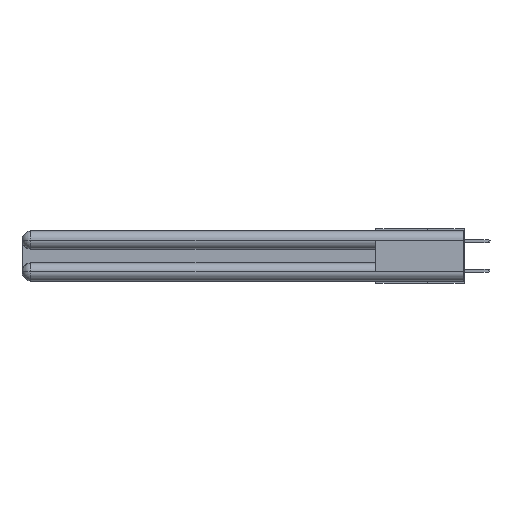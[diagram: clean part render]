
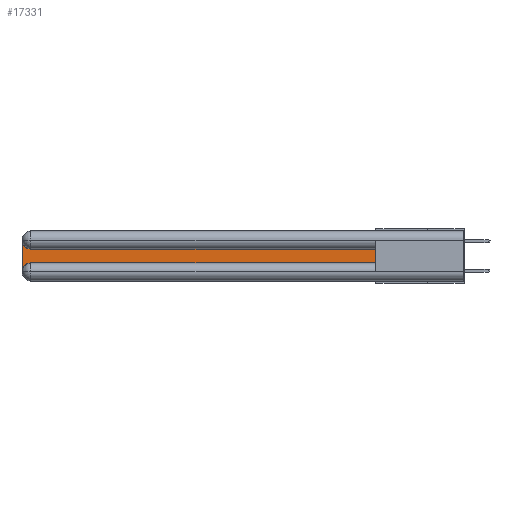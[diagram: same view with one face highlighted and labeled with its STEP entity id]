
A CAD part, left-side view. The second image highlights one B-rep face of the part: STEP entity #17331.
In plain terms, the highlighted planar face has unit normal (-1, 0, 0).
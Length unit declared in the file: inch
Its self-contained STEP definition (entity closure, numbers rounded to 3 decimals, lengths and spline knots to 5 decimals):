
#219 = CARTESIAN_POINT ( 'NONE',  ( 0.075, 3., -0.2775 ) ) ;
#752 = ORIENTED_EDGE ( 'NONE', *, *, #14818, .T. ) ;
#856 = CARTESIAN_POINT ( 'NONE',  ( 0.075, 3., -0.2175 ) ) ;
#1211 = VERTEX_POINT ( 'NONE', #23241 ) ;
#3234 = ORIENTED_EDGE ( 'NONE', *, *, #20636, .T. ) ;
#3417 = CARTESIAN_POINT ( 'NONE',  ( 0.075, 3., -0.0625 ) ) ;
#3495 = LINE ( 'NONE', #5955, #17714 ) ;
#3591 = PLANE ( 'NONE',  #27706 ) ;
#3923 = DIRECTION ( 'NONE',  ( 0., 0., -1. ) ) ;
#4102 = ORIENTED_EDGE ( 'NONE', *, *, #30607, .T. ) ;
#5374 = VECTOR ( 'NONE', #17422, 39.37008 ) ;
#5948 = DIRECTION ( 'NONE',  ( 0., 0., -1. ) ) ;
#5955 = CARTESIAN_POINT ( 'NONE',  ( 0.075, 0.6, -0.2175 ) ) ;
#6146 = CARTESIAN_POINT ( 'NONE',  ( 0.075, 3., -0.1225 ) ) ;
#6743 = CIRCLE ( 'NONE', #29178, 0.06 ) ;
#6991 = ORIENTED_EDGE ( 'NONE', *, *, #27049, .T. ) ;
#8334 = DIRECTION ( 'NONE',  ( 0., 0., -1. ) ) ;
#8492 = DIRECTION ( 'NONE',  ( 0., -1., 0. ) ) ;
#9001 = LINE ( 'NONE', #856, #20772 ) ;
#9965 = CARTESIAN_POINT ( 'NONE',  ( 0.075, 2.94, -0.2175 ) ) ;
#10862 = DIRECTION ( 'NONE',  ( 1., 0., 0. ) ) ;
#11037 = LINE ( 'NONE', #15248, #21231 ) ;
#14589 = CARTESIAN_POINT ( 'NONE',  ( 0.075, 0.6, -0.2175 ) ) ;
#14818 = EDGE_CURVE ( 'NONE', #27505, #26355, #6743, .T. ) ;
#15125 = DIRECTION ( 'NONE',  ( 0., 1., 0. ) ) ;
#15248 = CARTESIAN_POINT ( 'NONE',  ( 0.075, 0.6, -0.1225 ) ) ;
#15680 = EDGE_LOOP ( 'NONE', ( #20728, #4102, #3234, #752, #6991, #26406 ) ) ;
#17156 = CIRCLE ( 'NONE', #19850, 0.06 ) ;
#17331 = ADVANCED_FACE ( 'NONE', ( #25394 ), #3591, .F. ) ;
#17422 = DIRECTION ( 'NONE',  ( 0., 0., 1. ) ) ;
#17714 = VECTOR ( 'NONE', #8492, 39.37008 ) ;
#17903 = VERTEX_POINT ( 'NONE', #3417 ) ;
#19077 = CARTESIAN_POINT ( 'NONE',  ( 0.075, 2.94, -0.1225 ) ) ;
#19850 = AXIS2_PLACEMENT_3D ( 'NONE', #31209, #10862, #26201 ) ;
#19852 = CARTESIAN_POINT ( 'NONE',  ( 0.075, 0.6, -0.2175 ) ) ;
#20636 = EDGE_CURVE ( 'NONE', #17903, #27505, #9001, .T. ) ;
#20728 = ORIENTED_EDGE ( 'NONE', *, *, #28156, .T. ) ;
#20744 = DIRECTION ( 'NONE',  ( 1., 0., 0. ) ) ;
#20772 = VECTOR ( 'NONE', #5948, 39.37008 ) ;
#21231 = VECTOR ( 'NONE', #15125, 39.37008 ) ;
#21952 = LINE ( 'NONE', #19852, #5374 ) ;
#23054 = VERTEX_POINT ( 'NONE', #14589 ) ;
#23241 = CARTESIAN_POINT ( 'NONE',  ( 0.075, 0.6, -0.1225 ) ) ;
#25394 = FACE_OUTER_BOUND ( 'NONE', #15680, .T. ) ;
#26201 = DIRECTION ( 'NONE',  ( 0., 0., -1. ) ) ;
#26258 = DIRECTION ( 'NONE',  ( 1., 0., 0. ) ) ;
#26355 = VERTEX_POINT ( 'NONE', #9965 ) ;
#26406 = ORIENTED_EDGE ( 'NONE', *, *, #29418, .T. ) ;
#27049 = EDGE_CURVE ( 'NONE', #26355, #23054, #3495, .T. ) ;
#27505 = VERTEX_POINT ( 'NONE', #219 ) ;
#27706 = AXIS2_PLACEMENT_3D ( 'NONE', #6146, #26258, #3923 ) ;
#28156 = EDGE_CURVE ( 'NONE', #1211, #28575, #11037, .T. ) ;
#28575 = VERTEX_POINT ( 'NONE', #19077 ) ;
#29178 = AXIS2_PLACEMENT_3D ( 'NONE', #30584, #20744, #8334 ) ;
#29418 = EDGE_CURVE ( 'NONE', #23054, #1211, #21952, .T. ) ;
#30584 = CARTESIAN_POINT ( 'NONE',  ( 0.075, 2.94, -0.2775 ) ) ;
#30607 = EDGE_CURVE ( 'NONE', #28575, #17903, #17156, .T. ) ;
#31209 = CARTESIAN_POINT ( 'NONE',  ( 0.075, 2.94, -0.0625 ) ) ;
